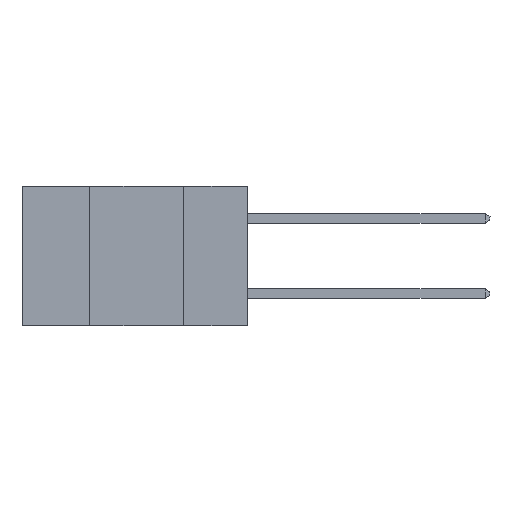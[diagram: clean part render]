
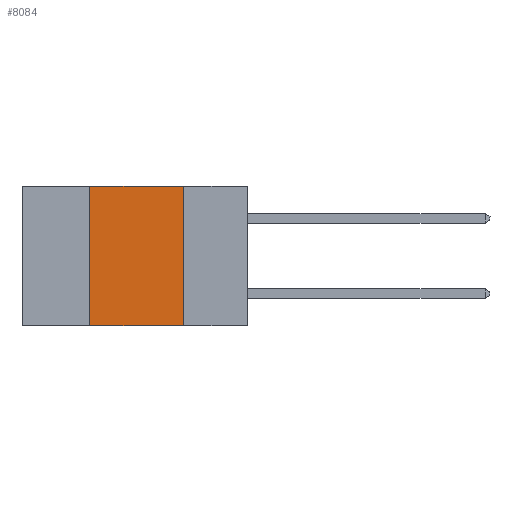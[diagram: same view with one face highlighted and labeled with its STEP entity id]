
A CAD part, left-side view. The second image highlights one B-rep face of the part: STEP entity #8084.
In plain terms, the highlighted planar face has unit normal (-1, 0, 0).
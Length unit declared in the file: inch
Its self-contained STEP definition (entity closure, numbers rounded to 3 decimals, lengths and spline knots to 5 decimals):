
#91 = VERTEX_POINT ( 'NONE', #2913 ) ;
#105 = EDGE_CURVE ( 'NONE', #91, #5281, #1438, .T. ) ;
#235 = FACE_OUTER_BOUND ( 'NONE', #1445, .T. ) ;
#477 = EDGE_CURVE ( 'NONE', #6206, #91, #3932, .T. ) ;
#1099 = ORIENTED_EDGE ( 'NONE', *, *, #7411, .F. ) ;
#1438 = LINE ( 'NONE', #3437, #6834 ) ;
#1445 = EDGE_LOOP ( 'NONE', ( #1099, #4449, #7503, #1942 ) ) ;
#1807 = CARTESIAN_POINT ( 'NONE',  ( 0., 0.42, -0.37 ) ) ;
#1942 = ORIENTED_EDGE ( 'NONE', *, *, #8345, .T. ) ;
#2310 = VECTOR ( 'NONE', #4018, 39.37008 ) ;
#2438 = CARTESIAN_POINT ( 'NONE',  ( 0., 0.17, 0. ) ) ;
#2806 = DIRECTION ( 'NONE',  ( 0., -1., 0. ) ) ;
#2913 = CARTESIAN_POINT ( 'NONE',  ( 0., 0.42, 0. ) ) ;
#3253 = CARTESIAN_POINT ( 'NONE',  ( 0., 0.42, -0.37 ) ) ;
#3264 = VECTOR ( 'NONE', #7880, 39.37008 ) ;
#3437 = CARTESIAN_POINT ( 'NONE',  ( 0., 0.6, 0. ) ) ;
#3641 = CARTESIAN_POINT ( 'NONE',  ( 0., 0.17, -0.37 ) ) ;
#3932 = LINE ( 'NONE', #3253, #3264 ) ;
#4018 = DIRECTION ( 'NONE',  ( 0., 0., -1. ) ) ;
#4125 = CARTESIAN_POINT ( 'NONE',  ( 0., 0.6, -0.37 ) ) ;
#4239 = PLANE ( 'NONE',  #6843 ) ;
#4431 = VERTEX_POINT ( 'NONE', #3641 ) ;
#4449 = ORIENTED_EDGE ( 'NONE', *, *, #105, .F. ) ;
#4766 = DIRECTION ( 'NONE',  ( 0., -1., 0. ) ) ;
#4967 = DIRECTION ( 'NONE',  ( 0., 0., -1. ) ) ;
#5281 = VERTEX_POINT ( 'NONE', #2438 ) ;
#5446 = VECTOR ( 'NONE', #2806, 39.37008 ) ;
#6126 = CARTESIAN_POINT ( 'NONE',  ( 0., 0.17, -0.37 ) ) ;
#6206 = VERTEX_POINT ( 'NONE', #1807 ) ;
#6214 = DIRECTION ( 'NONE',  ( 1., 0., 0. ) ) ;
#6790 = LINE ( 'NONE', #6126, #2310 ) ;
#6834 = VECTOR ( 'NONE', #4766, 39.37008 ) ;
#6843 = AXIS2_PLACEMENT_3D ( 'NONE', #6870, #6214, #4967 ) ;
#6870 = CARTESIAN_POINT ( 'NONE',  ( 0., 0.6, 0. ) ) ;
#7411 = EDGE_CURVE ( 'NONE', #5281, #4431, #6790, .T. ) ;
#7503 = ORIENTED_EDGE ( 'NONE', *, *, #477, .F. ) ;
#7880 = DIRECTION ( 'NONE',  ( 0., 0., 1. ) ) ;
#8062 = LINE ( 'NONE', #4125, #5446 ) ;
#8084 = ADVANCED_FACE ( 'NONE', ( #235 ), #4239, .F. ) ;
#8345 = EDGE_CURVE ( 'NONE', #6206, #4431, #8062, .T. ) ;
